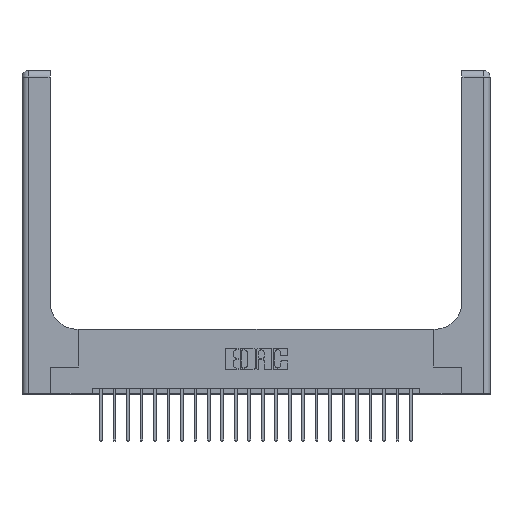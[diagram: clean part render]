
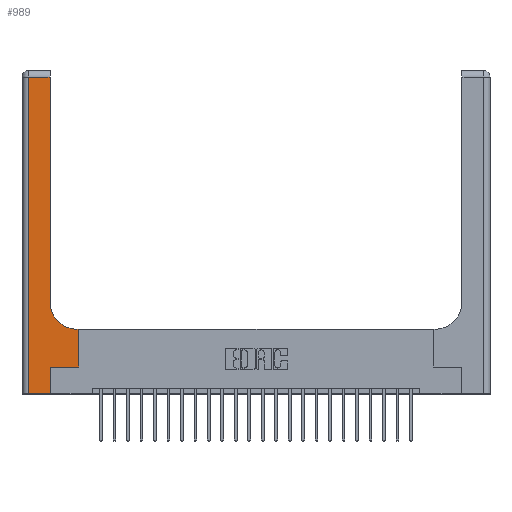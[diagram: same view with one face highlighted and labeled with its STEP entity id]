
A CAD part, top view. The second image highlights one B-rep face of the part: STEP entity #989.
In plain terms, the highlighted planar face has unit normal (0, 0, 1).
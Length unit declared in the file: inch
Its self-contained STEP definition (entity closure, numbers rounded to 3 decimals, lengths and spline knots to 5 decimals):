
#68 = EDGE_CURVE ( 'NONE', #19139, #2258, #7592, .T. ) ;
#236 = DIRECTION ( 'NONE',  ( 1., 0., 0. ) ) ;
#329 = VECTOR ( 'NONE', #1401, 39.37008 ) ;
#989 = ADVANCED_FACE ( 'NONE', ( #5193 ), #1236, .F. ) ;
#1236 = PLANE ( 'NONE',  #9814 ) ;
#1401 = DIRECTION ( 'NONE',  ( 1., 0., 0. ) ) ;
#2010 = DIRECTION ( 'NONE',  ( -1., 0., 0. ) ) ;
#2033 = DIRECTION ( 'NONE',  ( 0., 0., -1. ) ) ;
#2041 = LINE ( 'NONE', #5170, #11482 ) ;
#2095 = ORIENTED_EDGE ( 'NONE', *, *, #8315, .T. ) ;
#2258 = VERTEX_POINT ( 'NONE', #18015 ) ;
#2423 = CARTESIAN_POINT ( 'NONE',  ( 0.265, 0.25, 0.37 ) ) ;
#2481 = VECTOR ( 'NONE', #5907, 39.37008 ) ;
#3168 = LINE ( 'NONE', #5092, #9922 ) ;
#4837 = DIRECTION ( 'NONE',  ( 0., 0., -1. ) ) ;
#4857 = EDGE_CURVE ( 'NONE', #18935, #11534, #9146, .T. ) ;
#5092 = CARTESIAN_POINT ( 'NONE',  ( 0.528, 0.25, 0.37 ) ) ;
#5133 = EDGE_CURVE ( 'NONE', #20214, #17581, #19671, .T. ) ;
#5170 = CARTESIAN_POINT ( 'NONE',  ( 0., 2.94, 0.37 ) ) ;
#5193 = FACE_OUTER_BOUND ( 'NONE', #13955, .T. ) ;
#5793 = EDGE_CURVE ( 'NONE', #19291, #16163, #2041, .T. ) ;
#5907 = DIRECTION ( 'NONE',  ( 1., 0., 0. ) ) ;
#6120 = VECTOR ( 'NONE', #16857, 39.37008 ) ;
#6481 = ORIENTED_EDGE ( 'NONE', *, *, #13615, .T. ) ;
#6702 = ORIENTED_EDGE ( 'NONE', *, *, #13855, .T. ) ;
#7051 = CARTESIAN_POINT ( 'NONE',  ( 0., 0., 0.37 ) ) ;
#7215 = AXIS2_PLACEMENT_3D ( 'NONE', #7447, #2033, #236 ) ;
#7293 = ORIENTED_EDGE ( 'NONE', *, *, #5793, .T. ) ;
#7447 = CARTESIAN_POINT ( 'NONE',  ( 0.51, 0.85, 0.37 ) ) ;
#7592 = LINE ( 'NONE', #2423, #2481 ) ;
#8110 = CARTESIAN_POINT ( 'NONE',  ( 0.265, 0., 0.37 ) ) ;
#8315 = EDGE_CURVE ( 'NONE', #2258, #19668, #3168, .T. ) ;
#8570 = DIRECTION ( 'NONE',  ( -1., 0., 0. ) ) ;
#8842 = DIRECTION ( 'NONE',  ( 0., 1., 0. ) ) ;
#8918 = VECTOR ( 'NONE', #2010, 39.37008 ) ;
#9146 = CIRCLE ( 'NONE', #7215, 0.25 ) ;
#9814 = AXIS2_PLACEMENT_3D ( 'NONE', #14209, #4837, #8570 ) ;
#9913 = CARTESIAN_POINT ( 'NONE',  ( 0.06, 3., 0.37 ) ) ;
#9922 = VECTOR ( 'NONE', #10513, 39.37008 ) ;
#10044 = EDGE_CURVE ( 'NONE', #16163, #20214, #13870, .T. ) ;
#10227 = ORIENTED_EDGE ( 'NONE', *, *, #68, .T. ) ;
#10333 = EDGE_CURVE ( 'NONE', #11534, #19291, #13133, .T. ) ;
#10513 = DIRECTION ( 'NONE',  ( 0., 1., 0. ) ) ;
#11482 = VECTOR ( 'NONE', #18033, 39.37008 ) ;
#11534 = VERTEX_POINT ( 'NONE', #23116 ) ;
#13133 = LINE ( 'NONE', #14702, #6120 ) ;
#13615 = EDGE_CURVE ( 'NONE', #19668, #18935, #20514, .T. ) ;
#13855 = EDGE_CURVE ( 'NONE', #17581, #19139, #20387, .T. ) ;
#13870 = LINE ( 'NONE', #9913, #21102 ) ;
#13930 = VECTOR ( 'NONE', #8842, 39.37008 ) ;
#13955 = EDGE_LOOP ( 'NONE', ( #22888, #7293, #15786, #20623, #6702, #10227, #2095, #6481, #21508 ) ) ;
#14209 = CARTESIAN_POINT ( 'NONE',  ( 0., 3., 0.37 ) ) ;
#14702 = CARTESIAN_POINT ( 'NONE',  ( 0.26, 3., 0.37 ) ) ;
#15171 = CARTESIAN_POINT ( 'NONE',  ( 0.06, 2.94, 0.37 ) ) ;
#15786 = ORIENTED_EDGE ( 'NONE', *, *, #10044, .T. ) ;
#15788 = CARTESIAN_POINT ( 'NONE',  ( 0.528, 0.6, 0.37 ) ) ;
#16163 = VERTEX_POINT ( 'NONE', #15171 ) ;
#16315 = CARTESIAN_POINT ( 'NONE',  ( 0.26, 2.94, 0.37 ) ) ;
#16857 = DIRECTION ( 'NONE',  ( 0., 1., 0. ) ) ;
#17306 = CARTESIAN_POINT ( 'NONE',  ( 0.51, 0.6, 0.37 ) ) ;
#17581 = VERTEX_POINT ( 'NONE', #8110 ) ;
#18015 = CARTESIAN_POINT ( 'NONE',  ( 0.528, 0.25, 0.37 ) ) ;
#18033 = DIRECTION ( 'NONE',  ( -1., 0., 0. ) ) ;
#18477 = CARTESIAN_POINT ( 'NONE',  ( 0.26, 0.6, 0.37 ) ) ;
#18935 = VERTEX_POINT ( 'NONE', #17306 ) ;
#19139 = VERTEX_POINT ( 'NONE', #23281 ) ;
#19291 = VERTEX_POINT ( 'NONE', #16315 ) ;
#19668 = VERTEX_POINT ( 'NONE', #15788 ) ;
#19671 = LINE ( 'NONE', #7051, #329 ) ;
#20144 = CARTESIAN_POINT ( 'NONE',  ( 0.265, 0., 0.37 ) ) ;
#20214 = VERTEX_POINT ( 'NONE', #22434 ) ;
#20387 = LINE ( 'NONE', #20144, #13930 ) ;
#20514 = LINE ( 'NONE', #18477, #8918 ) ;
#20623 = ORIENTED_EDGE ( 'NONE', *, *, #5133, .T. ) ;
#20967 = DIRECTION ( 'NONE',  ( 0., -1., 0. ) ) ;
#21102 = VECTOR ( 'NONE', #20967, 39.37008 ) ;
#21508 = ORIENTED_EDGE ( 'NONE', *, *, #4857, .T. ) ;
#22434 = CARTESIAN_POINT ( 'NONE',  ( 0.06, 0., 0.37 ) ) ;
#22888 = ORIENTED_EDGE ( 'NONE', *, *, #10333, .T. ) ;
#23116 = CARTESIAN_POINT ( 'NONE',  ( 0.26, 0.85, 0.37 ) ) ;
#23281 = CARTESIAN_POINT ( 'NONE',  ( 0.265, 0.25, 0.37 ) ) ;
